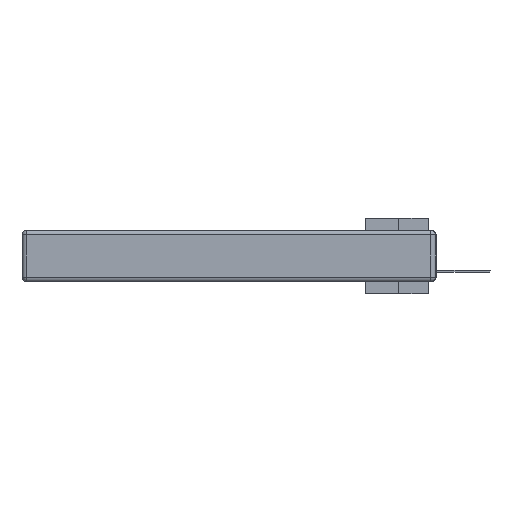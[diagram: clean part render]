
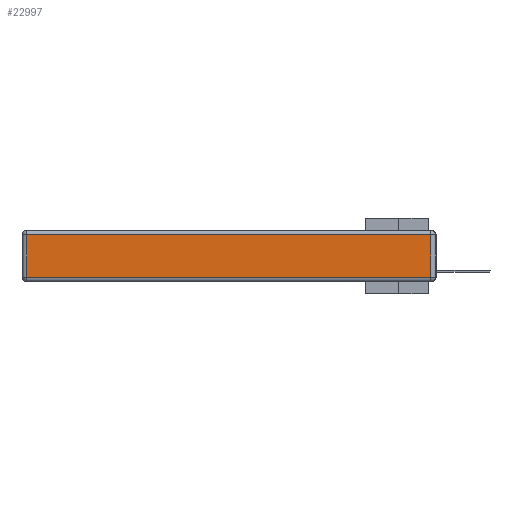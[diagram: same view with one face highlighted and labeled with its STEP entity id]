
A CAD part, left-side view. The second image highlights one B-rep face of the part: STEP entity #22997.
In plain terms, the highlighted planar face has unit normal (-1, 0, 0).
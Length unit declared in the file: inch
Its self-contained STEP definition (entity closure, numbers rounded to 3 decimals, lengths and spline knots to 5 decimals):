
#2703 = CARTESIAN_POINT ( 'NONE',  ( 0., 0.03, -0.343 ) ) ;
#2986 = VERTEX_POINT ( 'NONE', #32581 ) ;
#6997 = EDGE_CURVE ( 'NONE', #24993, #2986, #12065, .T. ) ;
#7335 = ORIENTED_EDGE ( 'NONE', *, *, #6997, .T. ) ;
#7800 = PLANE ( 'NONE',  #32296 ) ;
#8249 = DIRECTION ( 'NONE',  ( 0., 0., 1. ) ) ;
#9460 = FACE_OUTER_BOUND ( 'NONE', #27538, .T. ) ;
#9551 = EDGE_CURVE ( 'NONE', #2986, #24136, #27500, .T. ) ;
#11851 = VECTOR ( 'NONE', #21342, 39.37008 ) ;
#12065 = LINE ( 'NONE', #29798, #15042 ) ;
#13137 = CARTESIAN_POINT ( 'NONE',  ( 0., 2.72, -0.313 ) ) ;
#14926 = CARTESIAN_POINT ( 'NONE',  ( 0., 0.03, -0.03 ) ) ;
#15042 = VECTOR ( 'NONE', #32617, 39.37008 ) ;
#15989 = EDGE_CURVE ( 'NONE', #27724, #24993, #25410, .T. ) ;
#16411 = DIRECTION ( 'NONE',  ( -1., 0., 0. ) ) ;
#16565 = ORIENTED_EDGE ( 'NONE', *, *, #29937, .T. ) ;
#20290 = VECTOR ( 'NONE', #23391, 39.37008 ) ;
#20998 = ORIENTED_EDGE ( 'NONE', *, *, #15989, .T. ) ;
#21342 = DIRECTION ( 'NONE',  ( 0., 0., -1. ) ) ;
#22997 = ADVANCED_FACE ( 'NONE', ( #9460 ), #7800, .T. ) ;
#23391 = DIRECTION ( 'NONE',  ( 0., -1., 0. ) ) ;
#24136 = VERTEX_POINT ( 'NONE', #13137 ) ;
#24398 = CARTESIAN_POINT ( 'NONE',  ( 0., 2.72, -0.343 ) ) ;
#24993 = VERTEX_POINT ( 'NONE', #14926 ) ;
#25410 = LINE ( 'NONE', #2703, #27503 ) ;
#27429 = ORIENTED_EDGE ( 'NONE', *, *, #9551, .T. ) ;
#27500 = LINE ( 'NONE', #24398, #11851 ) ;
#27503 = VECTOR ( 'NONE', #27586, 39.37008 ) ;
#27538 = EDGE_LOOP ( 'NONE', ( #16565, #20998, #7335, #27429 ) ) ;
#27586 = DIRECTION ( 'NONE',  ( 0., 0., 1. ) ) ;
#27724 = VERTEX_POINT ( 'NONE', #29658 ) ;
#28319 = LINE ( 'NONE', #34334, #20290 ) ;
#29658 = CARTESIAN_POINT ( 'NONE',  ( 0., 0.03, -0.313 ) ) ;
#29798 = CARTESIAN_POINT ( 'NONE',  ( 0., 2.75, -0.03 ) ) ;
#29937 = EDGE_CURVE ( 'NONE', #24136, #27724, #28319, .T. ) ;
#30336 = CARTESIAN_POINT ( 'NONE',  ( 0., 0., -0.343 ) ) ;
#32296 = AXIS2_PLACEMENT_3D ( 'NONE', #30336, #16411, #8249 ) ;
#32581 = CARTESIAN_POINT ( 'NONE',  ( 0., 2.72, -0.03 ) ) ;
#32617 = DIRECTION ( 'NONE',  ( 0., 1., 0. ) ) ;
#34334 = CARTESIAN_POINT ( 'NONE',  ( 0., 0., -0.313 ) ) ;
